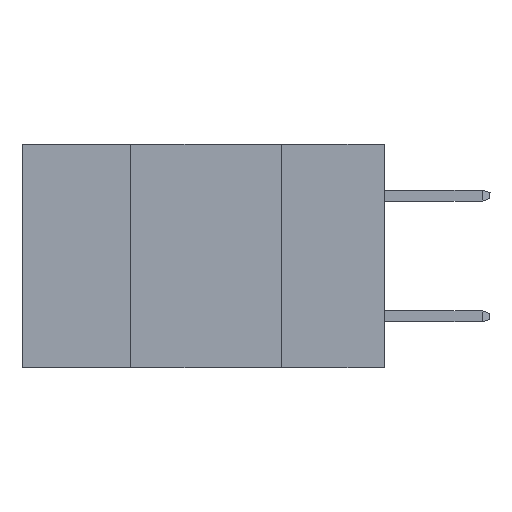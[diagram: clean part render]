
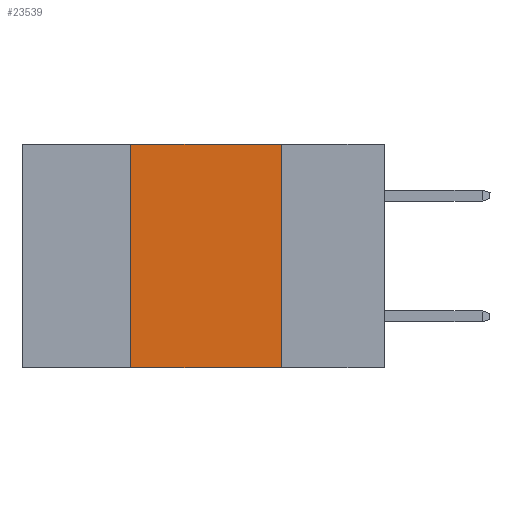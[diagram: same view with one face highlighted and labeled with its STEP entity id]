
A CAD part, left-side view. The second image highlights one B-rep face of the part: STEP entity #23539.
In plain terms, the highlighted planar face has unit normal (-1, 0, 0).
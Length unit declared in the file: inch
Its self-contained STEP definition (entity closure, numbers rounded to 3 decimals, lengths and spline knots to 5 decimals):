
#407 = CARTESIAN_POINT ( 'NONE',  ( 0., 0.17, 0. ) ) ;
#745 = VECTOR ( 'NONE', #24200, 39.37008 ) ;
#2153 = ORIENTED_EDGE ( 'NONE', *, *, #2177, .F. ) ;
#2177 = EDGE_CURVE ( 'NONE', #20991, #4525, #8126, .T. ) ;
#2244 = CARTESIAN_POINT ( 'NONE',  ( 0., 0.17, 0. ) ) ;
#3017 = EDGE_CURVE ( 'NONE', #13489, #17352, #26924, .T. ) ;
#3178 = CARTESIAN_POINT ( 'NONE',  ( 0., 0.42, 0. ) ) ;
#3269 = PLANE ( 'NONE',  #28238 ) ;
#4525 = VERTEX_POINT ( 'NONE', #14921 ) ;
#5571 = ORIENTED_EDGE ( 'NONE', *, *, #20506, .T. ) ;
#7470 = DIRECTION ( 'NONE',  ( 1., 0., 0. ) ) ;
#8126 = LINE ( 'NONE', #3178, #18101 ) ;
#12363 = DIRECTION ( 'NONE',  ( 0., -1., 0. ) ) ;
#13259 = VECTOR ( 'NONE', #24446, 39.37008 ) ;
#13294 = CARTESIAN_POINT ( 'NONE',  ( 0., 0.6, 0. ) ) ;
#13489 = VERTEX_POINT ( 'NONE', #407 ) ;
#14240 = EDGE_CURVE ( 'NONE', #4525, #13489, #22304, .T. ) ;
#14821 = CARTESIAN_POINT ( 'NONE',  ( 0., 0.17, -0.37 ) ) ;
#14921 = CARTESIAN_POINT ( 'NONE',  ( 0., 0.42, 0. ) ) ;
#15473 = ORIENTED_EDGE ( 'NONE', *, *, #3017, .F. ) ;
#16226 = DIRECTION ( 'NONE',  ( 0., 0., 1. ) ) ;
#17210 = LINE ( 'NONE', #25464, #28114 ) ;
#17352 = VERTEX_POINT ( 'NONE', #14821 ) ;
#18101 = VECTOR ( 'NONE', #16226, 39.37008 ) ;
#19261 = EDGE_LOOP ( 'NONE', ( #15473, #24302, #2153, #5571 ) ) ;
#19410 = FACE_OUTER_BOUND ( 'NONE', #19261, .T. ) ;
#20506 = EDGE_CURVE ( 'NONE', #20991, #17352, #17210, .T. ) ;
#20609 = CARTESIAN_POINT ( 'NONE',  ( 0., 0.6, 0. ) ) ;
#20991 = VERTEX_POINT ( 'NONE', #24539 ) ;
#22304 = LINE ( 'NONE', #13294, #745 ) ;
#22888 = DIRECTION ( 'NONE',  ( 0., 0., -1. ) ) ;
#23539 = ADVANCED_FACE ( 'NONE', ( #19410 ), #3269, .F. ) ;
#24200 = DIRECTION ( 'NONE',  ( 0., -1., 0. ) ) ;
#24302 = ORIENTED_EDGE ( 'NONE', *, *, #14240, .F. ) ;
#24446 = DIRECTION ( 'NONE',  ( 0., 0., -1. ) ) ;
#24539 = CARTESIAN_POINT ( 'NONE',  ( 0., 0.42, -0.37 ) ) ;
#25464 = CARTESIAN_POINT ( 'NONE',  ( 0., 0.6, -0.37 ) ) ;
#26924 = LINE ( 'NONE', #2244, #13259 ) ;
#28114 = VECTOR ( 'NONE', #12363, 39.37008 ) ;
#28238 = AXIS2_PLACEMENT_3D ( 'NONE', #20609, #7470, #22888 ) ;
